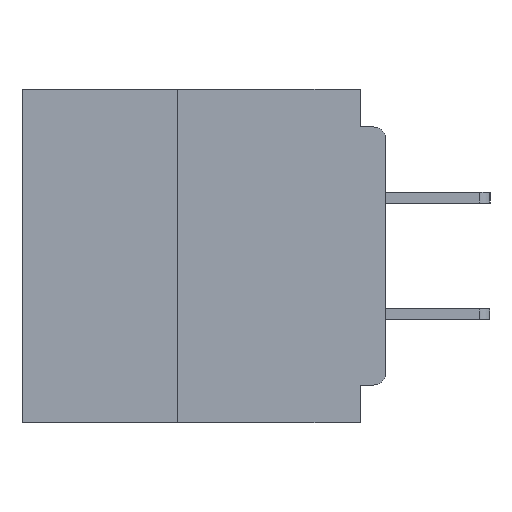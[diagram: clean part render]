
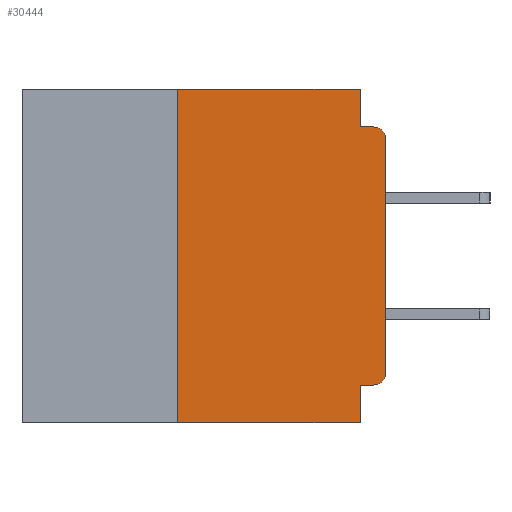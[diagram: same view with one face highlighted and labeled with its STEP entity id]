
A CAD part, left-side view. The second image highlights one B-rep face of the part: STEP entity #30444.
In plain terms, the highlighted planar face has unit normal (-1, 0, 0).
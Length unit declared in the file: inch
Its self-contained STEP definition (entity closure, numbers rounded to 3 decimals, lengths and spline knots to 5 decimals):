
#239 = DIRECTION ( 'NONE',  ( 0., -1., 0. ) ) ;
#324 = ORIENTED_EDGE ( 'NONE', *, *, #30688, .F. ) ;
#524 = CARTESIAN_POINT ( 'NONE',  ( 0., 0.015, -0.355 ) ) ;
#702 = VECTOR ( 'NONE', #239, 39.37008 ) ;
#758 = ORIENTED_EDGE ( 'NONE', *, *, #20788, .T. ) ;
#3059 = EDGE_CURVE ( 'NONE', #30691, #5805, #6544, .T. ) ;
#4478 = CARTESIAN_POINT ( 'NONE',  ( 0., 0.031, -0.4 ) ) ;
#5360 = LINE ( 'NONE', #18567, #34490 ) ;
#5805 = VERTEX_POINT ( 'NONE', #29227 ) ;
#5904 = DIRECTION ( 'NONE',  ( 0., 0., -1. ) ) ;
#6544 = LINE ( 'NONE', #33041, #33513 ) ;
#6710 = ORIENTED_EDGE ( 'NONE', *, *, #19204, .F. ) ;
#7686 = CARTESIAN_POINT ( 'NONE',  ( 0., 0., -0.045 ) ) ;
#7961 = EDGE_CURVE ( 'NONE', #17833, #43456, #33127, .T. ) ;
#9726 = CARTESIAN_POINT ( 'NONE',  ( 0., 0.031, 0. ) ) ;
#9953 = EDGE_CURVE ( 'NONE', #18633, #43456, #31278, .T. ) ;
#9988 = DIRECTION ( 'NONE',  ( -1., 0., 0. ) ) ;
#10481 = DIRECTION ( 'NONE',  ( 0., 0., 1. ) ) ;
#11251 = LINE ( 'NONE', #21180, #702 ) ;
#11415 = VERTEX_POINT ( 'NONE', #524 ) ;
#11442 = DIRECTION ( 'NONE',  ( 1., 0., 0. ) ) ;
#12733 = CIRCLE ( 'NONE', #31690, 0.015 ) ;
#13133 = DIRECTION ( 'NONE',  ( 0., 0., -1. ) ) ;
#14132 = CARTESIAN_POINT ( 'NONE',  ( 0., 0.015, -0.06 ) ) ;
#14255 = ORIENTED_EDGE ( 'NONE', *, *, #3059, .F. ) ;
#14474 = VECTOR ( 'NONE', #18311, 39.37008 ) ;
#16062 = CARTESIAN_POINT ( 'NONE',  ( 0., 0., -0.34 ) ) ;
#17513 = EDGE_CURVE ( 'NONE', #11415, #18760, #12733, .T. ) ;
#17637 = DIRECTION ( 'NONE',  ( 0., 0., -1. ) ) ;
#17708 = CARTESIAN_POINT ( 'NONE',  ( 0., 0., 0. ) ) ;
#17833 = VERTEX_POINT ( 'NONE', #29320 ) ;
#18311 = DIRECTION ( 'NONE',  ( 0., -1., 0. ) ) ;
#18567 = CARTESIAN_POINT ( 'NONE',  ( 0., 0., -0.355 ) ) ;
#18587 = VERTEX_POINT ( 'NONE', #4478 ) ;
#18633 = VERTEX_POINT ( 'NONE', #39765 ) ;
#18760 = VERTEX_POINT ( 'NONE', #16062 ) ;
#19204 = EDGE_CURVE ( 'NONE', #11415, #26329, #5360, .T. ) ;
#20275 = CARTESIAN_POINT ( 'NONE',  ( 0., 0.031, 0. ) ) ;
#20283 = CARTESIAN_POINT ( 'NONE',  ( 0., 0.25, -0.4 ) ) ;
#20788 = EDGE_CURVE ( 'NONE', #18760, #18633, #23345, .T. ) ;
#21180 = CARTESIAN_POINT ( 'NONE',  ( 0., 0.437, 0. ) ) ;
#22047 = CARTESIAN_POINT ( 'NONE',  ( 0., 0.437, -0.4 ) ) ;
#23345 = LINE ( 'NONE', #17708, #41909 ) ;
#23507 = LINE ( 'NONE', #22047, #40996 ) ;
#25604 = VECTOR ( 'NONE', #5904, 39.37008 ) ;
#25621 = DIRECTION ( 'NONE',  ( 0., -1., 0. ) ) ;
#26329 = VERTEX_POINT ( 'NONE', #31509 ) ;
#26950 = ORIENTED_EDGE ( 'NONE', *, *, #9953, .T. ) ;
#27039 = ORIENTED_EDGE ( 'NONE', *, *, #30076, .F. ) ;
#27805 = ORIENTED_EDGE ( 'NONE', *, *, #7961, .F. ) ;
#28283 = VECTOR ( 'NONE', #13133, 39.37008 ) ;
#28871 = FACE_OUTER_BOUND ( 'NONE', #30862, .T. ) ;
#29182 = VERTEX_POINT ( 'NONE', #20275 ) ;
#29227 = CARTESIAN_POINT ( 'NONE',  ( 0., 0.25, 0. ) ) ;
#29320 = CARTESIAN_POINT ( 'NONE',  ( 0., 0.031, -0.045 ) ) ;
#29432 = CARTESIAN_POINT ( 'NONE',  ( 0., 0.015, -0.045 ) ) ;
#30076 = EDGE_CURVE ( 'NONE', #26329, #18587, #34924, .T. ) ;
#30444 = ADVANCED_FACE ( 'NONE', ( #28871 ), #32312, .F. ) ;
#30688 = EDGE_CURVE ( 'NONE', #29182, #17833, #39747, .T. ) ;
#30691 = VERTEX_POINT ( 'NONE', #20283 ) ;
#30862 = EDGE_LOOP ( 'NONE', ( #758, #26950, #27805, #324, #45249, #14255, #36499, #27039, #6710, #40238 ) ) ;
#30889 = EDGE_CURVE ( 'NONE', #5805, #29182, #11251, .T. ) ;
#31035 = CARTESIAN_POINT ( 'NONE',  ( 0., 0.015, -0.34 ) ) ;
#31278 = CIRCLE ( 'NONE', #41540, 0.015 ) ;
#31509 = CARTESIAN_POINT ( 'NONE',  ( 0., 0.031, -0.355 ) ) ;
#31690 = AXIS2_PLACEMENT_3D ( 'NONE', #31035, #9988, #34539 ) ;
#32312 = PLANE ( 'NONE',  #45105 ) ;
#32375 = DIRECTION ( 'NONE',  ( 0., 0., 1. ) ) ;
#32462 = CARTESIAN_POINT ( 'NONE',  ( 0., 0.437, 0. ) ) ;
#33041 = CARTESIAN_POINT ( 'NONE',  ( 0., 0.25, -0.4 ) ) ;
#33127 = LINE ( 'NONE', #7686, #14474 ) ;
#33513 = VECTOR ( 'NONE', #32375, 39.37008 ) ;
#34490 = VECTOR ( 'NONE', #43015, 39.37008 ) ;
#34539 = DIRECTION ( 'NONE',  ( 0., 0., -1. ) ) ;
#34924 = LINE ( 'NONE', #37374, #25604 ) ;
#34973 = EDGE_CURVE ( 'NONE', #30691, #18587, #23507, .T. ) ;
#35971 = DIRECTION ( 'NONE',  ( 0., 0., -1. ) ) ;
#36499 = ORIENTED_EDGE ( 'NONE', *, *, #34973, .T. ) ;
#37374 = CARTESIAN_POINT ( 'NONE',  ( 0., 0.031, -0.4 ) ) ;
#38588 = DIRECTION ( 'NONE',  ( -1., 0., 0. ) ) ;
#39747 = LINE ( 'NONE', #9726, #28283 ) ;
#39765 = CARTESIAN_POINT ( 'NONE',  ( 0., 0., -0.06 ) ) ;
#40238 = ORIENTED_EDGE ( 'NONE', *, *, #17513, .T. ) ;
#40996 = VECTOR ( 'NONE', #25621, 39.37008 ) ;
#41540 = AXIS2_PLACEMENT_3D ( 'NONE', #14132, #38588, #17637 ) ;
#41909 = VECTOR ( 'NONE', #10481, 39.37008 ) ;
#43015 = DIRECTION ( 'NONE',  ( 0., 1., 0. ) ) ;
#43456 = VERTEX_POINT ( 'NONE', #29432 ) ;
#45105 = AXIS2_PLACEMENT_3D ( 'NONE', #32462, #11442, #35971 ) ;
#45249 = ORIENTED_EDGE ( 'NONE', *, *, #30889, .F. ) ;
